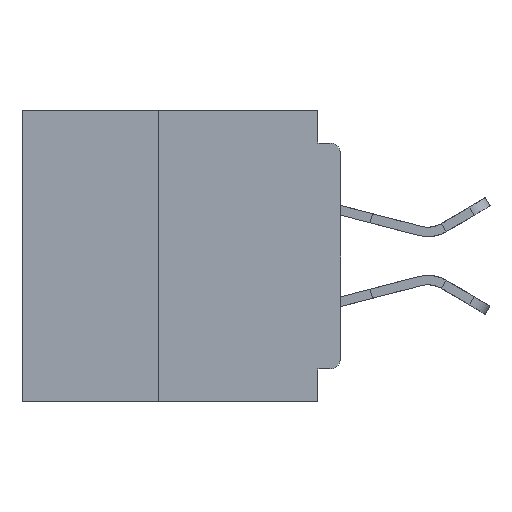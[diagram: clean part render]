
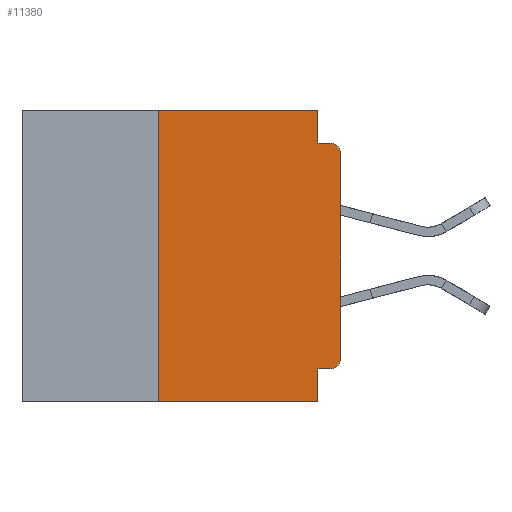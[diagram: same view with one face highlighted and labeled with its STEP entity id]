
A CAD part, left-side view. The second image highlights one B-rep face of the part: STEP entity #11380.
In plain terms, the highlighted planar face has unit normal (-1, 0, 0).
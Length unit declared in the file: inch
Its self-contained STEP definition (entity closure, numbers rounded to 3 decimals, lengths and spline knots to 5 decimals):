
#145 = DIRECTION ( 'NONE',  ( 0., -1., 0. ) ) ;
#364 = VECTOR ( 'NONE', #12365, 39.37008 ) ;
#714 = VECTOR ( 'NONE', #2715, 39.37008 ) ;
#1498 = CARTESIAN_POINT ( 'NONE',  ( 0., 0.015, -0.045 ) ) ;
#2715 = DIRECTION ( 'NONE',  ( 0., -1., 0. ) ) ;
#3791 = EDGE_CURVE ( 'NONE', #26153, #5124, #29301, .T. ) ;
#4474 = VERTEX_POINT ( 'NONE', #35661 ) ;
#4617 = EDGE_LOOP ( 'NONE', ( #30161, #11000, #8822, #22298, #16991, #36551, #11446, #10044, #11448, #10688 ) ) ;
#4934 = EDGE_CURVE ( 'NONE', #47865, #29929, #47112, .T. ) ;
#5054 = LINE ( 'NONE', #39504, #43363 ) ;
#5124 = VERTEX_POINT ( 'NONE', #39297 ) ;
#5653 = VERTEX_POINT ( 'NONE', #13510 ) ;
#5672 = VECTOR ( 'NONE', #17651, 39.37008 ) ;
#6010 = DIRECTION ( 'NONE',  ( 1., 0., 0. ) ) ;
#6237 = CARTESIAN_POINT ( 'NONE',  ( 0., 0.25, -0.4 ) ) ;
#6861 = LINE ( 'NONE', #36142, #5672 ) ;
#7845 = CARTESIAN_POINT ( 'NONE',  ( 0., 0., -0.06 ) ) ;
#8240 = EDGE_CURVE ( 'NONE', #4474, #26624, #19645, .T. ) ;
#8636 = CARTESIAN_POINT ( 'NONE',  ( 0., 0., 0. ) ) ;
#8822 = ORIENTED_EDGE ( 'NONE', *, *, #29885, .F. ) ;
#9622 = CARTESIAN_POINT ( 'NONE',  ( 0., 0.437, 0. ) ) ;
#10044 = ORIENTED_EDGE ( 'NONE', *, *, #39818, .F. ) ;
#10688 = ORIENTED_EDGE ( 'NONE', *, *, #8240, .T. ) ;
#11000 = ORIENTED_EDGE ( 'NONE', *, *, #4934, .T. ) ;
#11325 = LINE ( 'NONE', #33747, #28739 ) ;
#11380 = ADVANCED_FACE ( 'NONE', ( #43237 ), #31852, .F. ) ;
#11425 = AXIS2_PLACEMENT_3D ( 'NONE', #14316, #40224, #18022 ) ;
#11446 = ORIENTED_EDGE ( 'NONE', *, *, #41247, .T. ) ;
#11448 = ORIENTED_EDGE ( 'NONE', *, *, #46996, .F. ) ;
#11635 = AXIS2_PLACEMENT_3D ( 'NONE', #38196, #16011, #41923 ) ;
#11905 = CARTESIAN_POINT ( 'NONE',  ( 0., 0.25, 0. ) ) ;
#12365 = DIRECTION ( 'NONE',  ( 0., 0., 1. ) ) ;
#13510 = CARTESIAN_POINT ( 'NONE',  ( 0., 0.031, -0.355 ) ) ;
#13852 = EDGE_CURVE ( 'NONE', #35279, #26153, #32580, .T. ) ;
#14316 = CARTESIAN_POINT ( 'NONE',  ( 0., 0.015, -0.34 ) ) ;
#14627 = VECTOR ( 'NONE', #30488, 39.37008 ) ;
#15561 = CARTESIAN_POINT ( 'NONE',  ( 0., 0.031, 0. ) ) ;
#15909 = DIRECTION ( 'NONE',  ( 0., 0., 1. ) ) ;
#16011 = DIRECTION ( 'NONE',  ( -1., 0., 0. ) ) ;
#16991 = ORIENTED_EDGE ( 'NONE', *, *, #3791, .F. ) ;
#17651 = DIRECTION ( 'NONE',  ( 0., 1., 0. ) ) ;
#18022 = DIRECTION ( 'NONE',  ( 0., 0., -1. ) ) ;
#18696 = CARTESIAN_POINT ( 'NONE',  ( 0., 0., -0.34 ) ) ;
#19645 = CIRCLE ( 'NONE', #11425, 0.015 ) ;
#19853 = CARTESIAN_POINT ( 'NONE',  ( 0., 0.031, -0.4 ) ) ;
#20272 = LINE ( 'NONE', #8636, #364 ) ;
#22298 = ORIENTED_EDGE ( 'NONE', *, *, #39537, .F. ) ;
#23682 = CARTESIAN_POINT ( 'NONE',  ( 0., 0., -0.045 ) ) ;
#24437 = LINE ( 'NONE', #15561, #14627 ) ;
#24616 = CARTESIAN_POINT ( 'NONE',  ( 0., 0.031, -0.045 ) ) ;
#26098 = AXIS2_PLACEMENT_3D ( 'NONE', #9622, #6010, #32002 ) ;
#26153 = VERTEX_POINT ( 'NONE', #11905 ) ;
#26257 = VERTEX_POINT ( 'NONE', #19853 ) ;
#26624 = VERTEX_POINT ( 'NONE', #18696 ) ;
#27441 = DIRECTION ( 'NONE',  ( 0., -1., 0. ) ) ;
#28739 = VECTOR ( 'NONE', #145, 39.37008 ) ;
#28784 = CARTESIAN_POINT ( 'NONE',  ( 0., 0.437, 0. ) ) ;
#29301 = LINE ( 'NONE', #28784, #714 ) ;
#29885 = EDGE_CURVE ( 'NONE', #30085, #29929, #47651, .T. ) ;
#29929 = VERTEX_POINT ( 'NONE', #1498 ) ;
#30085 = VERTEX_POINT ( 'NONE', #24616 ) ;
#30161 = ORIENTED_EDGE ( 'NONE', *, *, #31668, .T. ) ;
#30488 = DIRECTION ( 'NONE',  ( 0., 0., -1. ) ) ;
#31668 = EDGE_CURVE ( 'NONE', #26624, #47865, #20272, .T. ) ;
#31852 = PLANE ( 'NONE',  #26098 ) ;
#32002 = DIRECTION ( 'NONE',  ( 0., 0., -1. ) ) ;
#32580 = LINE ( 'NONE', #38099, #43550 ) ;
#33747 = CARTESIAN_POINT ( 'NONE',  ( 0., 0.437, -0.4 ) ) ;
#35279 = VERTEX_POINT ( 'NONE', #6237 ) ;
#35661 = CARTESIAN_POINT ( 'NONE',  ( 0., 0.015, -0.355 ) ) ;
#35810 = DIRECTION ( 'NONE',  ( 0., 0., -1. ) ) ;
#36142 = CARTESIAN_POINT ( 'NONE',  ( 0., 0., -0.355 ) ) ;
#36551 = ORIENTED_EDGE ( 'NONE', *, *, #13852, .F. ) ;
#38099 = CARTESIAN_POINT ( 'NONE',  ( 0., 0.25, -0.4 ) ) ;
#38196 = CARTESIAN_POINT ( 'NONE',  ( 0., 0.015, -0.06 ) ) ;
#39297 = CARTESIAN_POINT ( 'NONE',  ( 0., 0.031, 0. ) ) ;
#39504 = CARTESIAN_POINT ( 'NONE',  ( 0., 0.031, -0.4 ) ) ;
#39537 = EDGE_CURVE ( 'NONE', #5124, #30085, #24437, .T. ) ;
#39818 = EDGE_CURVE ( 'NONE', #5653, #26257, #5054, .T. ) ;
#40224 = DIRECTION ( 'NONE',  ( -1., 0., 0. ) ) ;
#41247 = EDGE_CURVE ( 'NONE', #35279, #26257, #11325, .T. ) ;
#41923 = DIRECTION ( 'NONE',  ( 0., 0., -1. ) ) ;
#43237 = FACE_OUTER_BOUND ( 'NONE', #4617, .T. ) ;
#43363 = VECTOR ( 'NONE', #35810, 39.37008 ) ;
#43550 = VECTOR ( 'NONE', #15909, 39.37008 ) ;
#45340 = VECTOR ( 'NONE', #27441, 39.37008 ) ;
#46996 = EDGE_CURVE ( 'NONE', #4474, #5653, #6861, .T. ) ;
#47112 = CIRCLE ( 'NONE', #11635, 0.015 ) ;
#47651 = LINE ( 'NONE', #23682, #45340 ) ;
#47865 = VERTEX_POINT ( 'NONE', #7845 ) ;
